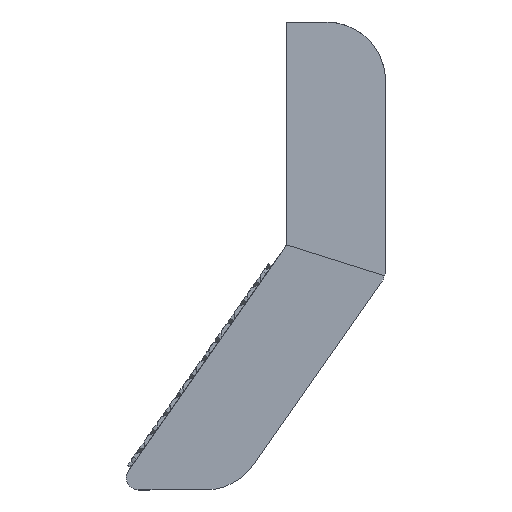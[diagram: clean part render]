
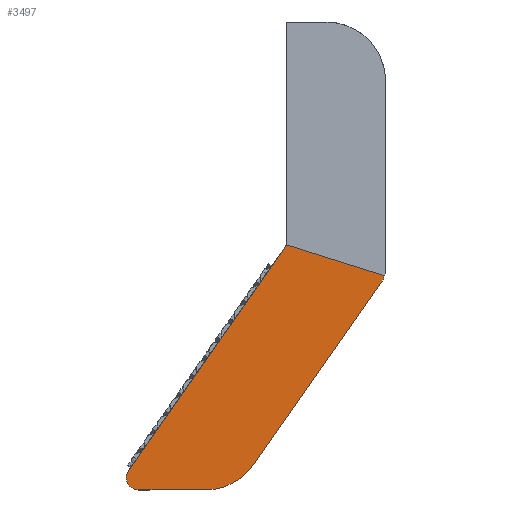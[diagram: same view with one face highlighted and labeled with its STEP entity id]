
A CAD part, left-side view. The second image highlights one B-rep face of the part: STEP entity #3497.
In plain terms, the highlighted planar face has unit normal (-0.999, -0.033, -0.023).
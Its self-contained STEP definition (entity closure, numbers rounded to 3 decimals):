
#36 = EDGE_CURVE ( 'NONE', #13042, #13123, #3158, .T. ) ;
#691 = CARTESIAN_POINT ( 'NONE',  ( -8.89, -15.225, -41.361 ) ) ;
#1274 = CARTESIAN_POINT ( 'NONE',  ( -9.399, 23.577, -74.676 ) ) ;
#1341 = DIRECTION ( 'NONE',  ( 0.033, -0.999, 0. ) ) ;
#1362 = CARTESIAN_POINT ( 'NONE',  ( -8.89, -15.225, -41.361 ) ) ;
#1385 = ORIENTED_EDGE ( 'NONE', *, *, #15113, .F. ) ;
#1728 = CARTESIAN_POINT ( 'NONE',  ( -9.525, 0.061, -35.626 ) ) ;
#1875 = ORIENTED_EDGE ( 'NONE', *, *, #10678, .F. ) ;
#1987 = LINE ( 'NONE', #13367, #2442 ) ;
#2082 = CARTESIAN_POINT ( 'NONE',  ( -9.399, 23.577, -74.676 ) ) ;
#2291 = VERTEX_POINT ( 'NONE', #15675 ) ;
#2442 = VECTOR ( 'NONE', #5008, 1000. ) ;
#2484 = EDGE_CURVE ( 'NONE', #17424, #4694, #1987, .T. ) ;
#2653 = CARTESIAN_POINT ( 'NONE',  ( -9.526, 0.037, -35.548 ) ) ;
#3158 =( BOUNDED_CURVE ( )  B_SPLINE_CURVE ( 3, ( #10948, #3732, #11009, #691 ),
 .UNSPECIFIED., .F., .F. ) 
 B_SPLINE_CURVE_WITH_KNOTS ( ( 4, 4 ),
 ( 5.978, 6.283 ),
 .UNSPECIFIED. ) 
 CURVE ( )  GEOMETRIC_REPRESENTATION_ITEM ( )  RATIONAL_B_SPLINE_CURVE ( ( 1., 0.992, 0.992, 1. ) ) 
 REPRESENTATION_ITEM ( '' )  );
#3220 = CARTESIAN_POINT ( 'NONE',  ( -9.399, 23.577, -74.676 ) ) ;
#3497 = ADVANCED_FACE ( 'NONE', ( #8715 ), #5661, .F. ) ;
#3581 = CARTESIAN_POINT ( 'NONE',  ( -9.46, 25.408, -74.676 ) ) ;
#3732 = CARTESIAN_POINT ( 'NONE',  ( -8.892, -15.554, -40.805 ) ) ;
#4188 = DIRECTION ( 'NONE',  ( 0.999, 0.033, 0.023 ) ) ;
#4454 = ORIENTED_EDGE ( 'NONE', *, *, #5288, .F. ) ;
#4624 =( BOUNDED_CURVE ( )  B_SPLINE_CURVE ( 3, ( #2082, #3581, #16139, #8078 ),
 .UNSPECIFIED., .F., .T. ) 
 B_SPLINE_CURVE_WITH_KNOTS ( ( 4, 4 ),
 ( 0.96, 3.142 ),
 .UNSPECIFIED. ) 
 CURVE ( )  GEOMETRIC_REPRESENTATION_ITEM ( )  RATIONAL_B_SPLINE_CURVE ( ( 1., 0.641, 0.641, 1. ) ) 
 REPRESENTATION_ITEM ( '' )  );
#4694 = VERTEX_POINT ( 'NONE', #5627 ) ;
#4769 = CARTESIAN_POINT ( 'NONE',  ( -9.525, 0.144, -35.765 ) ) ;
#5008 = DIRECTION ( 'NONE',  ( 0., 0.574, -0.819 ) ) ;
#5288 = EDGE_CURVE ( 'NONE', #9492, #13042, #16224, .T. ) ;
#5366 = CARTESIAN_POINT ( 'NONE',  ( -8.89, -15.225, -41.361 ) ) ;
#5627 = CARTESIAN_POINT ( 'NONE',  ( -9.525, 25.203, -71.553 ) ) ;
#5661 = PLANE ( 'NONE',  #12660 ) ;
#6237 = LINE ( 'NONE', #1274, #16676 ) ;
#6323 = CARTESIAN_POINT ( 'NONE',  ( -9.525, 0.144, -35.765 ) ) ;
#6362 = ORIENTED_EDGE ( 'NONE', *, *, #36, .F. ) ;
#6840 = CARTESIAN_POINT ( 'NONE',  ( -8.89, 5.259, -70.614 ) ) ;
#6990 = VECTOR ( 'NONE', #8749, 1000. ) ;
#6991 = EDGE_LOOP ( 'NONE', ( #4454, #12039, #12444, #1385, #9254, #1875, #13267, #6362 ) ) ;
#8078 = CARTESIAN_POINT ( 'NONE',  ( -9.525, 25.203, -71.553 ) ) ;
#8273 = CARTESIAN_POINT ( 'NONE',  ( -8.949, 9.89, -74.676 ) ) ;
#8715 = FACE_OUTER_BOUND ( 'NONE', #6991, .T. ) ;
#8749 = DIRECTION ( 'NONE',  ( 0., 0.574, -0.819 ) ) ;
#8948 = EDGE_CURVE ( 'NONE', #9492, #17424, #9407, .T. ) ;
#9254 = ORIENTED_EDGE ( 'NONE', *, *, #12468, .T. ) ;
#9407 =( BOUNDED_CURVE ( )  B_SPLINE_CURVE ( 3, ( #13176, #1728, #17095, #4769 ),
 .UNSPECIFIED., .F., .T. ) 
 B_SPLINE_CURVE_WITH_KNOTS ( ( 4, 4 ),
 ( 2.836, 3.142 ),
 .UNSPECIFIED. ) 
 CURVE ( )  GEOMETRIC_REPRESENTATION_ITEM ( )  RATIONAL_B_SPLINE_CURVE ( ( 1., 0.992, 0.992, 1. ) ) 
 REPRESENTATION_ITEM ( '' )  );
#9492 = VERTEX_POINT ( 'NONE', #15401 ) ;
#9546 = VECTOR ( 'NONE', #12680, 1000. ) ;
#10678 = EDGE_CURVE ( 'NONE', #2291, #13889, #14879, .T. ) ;
#10948 = CARTESIAN_POINT ( 'NONE',  ( -8.896, -15.652, -40.495 ) ) ;
#11009 = CARTESIAN_POINT ( 'NONE',  ( -8.89, -15.411, -41.096 ) ) ;
#11164 = LINE ( 'NONE', #1362, #6990 ) ;
#12039 = ORIENTED_EDGE ( 'NONE', *, *, #8948, .T. ) ;
#12444 = ORIENTED_EDGE ( 'NONE', *, *, #2484, .T. ) ;
#12468 = EDGE_CURVE ( 'NONE', #16759, #13889, #6237, .T. ) ;
#12660 = AXIS2_PLACEMENT_3D ( 'NONE', #16605, #4188, #14001 ) ;
#12680 = DIRECTION ( 'NONE',  ( 0.038, -0.953, -0.3 ) ) ;
#13042 = VERTEX_POINT ( 'NONE', #17567 ) ;
#13123 = VERTEX_POINT ( 'NONE', #5366 ) ;
#13176 = CARTESIAN_POINT ( 'NONE',  ( -9.526, 0.037, -35.548 ) ) ;
#13267 = ORIENTED_EDGE ( 'NONE', *, *, #14699, .F. ) ;
#13367 = CARTESIAN_POINT ( 'NONE',  ( -9.525, 0., -35.56 ) ) ;
#13655 = CARTESIAN_POINT ( 'NONE',  ( -8.89, 7.077, -73.212 ) ) ;
#13889 = VERTEX_POINT ( 'NONE', #17073 ) ;
#14001 = DIRECTION ( 'NONE',  ( -0.033, 0.999, 0. ) ) ;
#14699 = EDGE_CURVE ( 'NONE', #13123, #2291, #11164, .T. ) ;
#14879 =( BOUNDED_CURVE ( )  B_SPLINE_CURVE ( 3, ( #6840, #13655, #8273, #17651 ),
 .UNSPECIFIED., .F., .T. ) 
 B_SPLINE_CURVE_WITH_KNOTS ( ( 4, 4 ),
 ( 0., 0.96 ),
 .UNSPECIFIED. ) 
 CURVE ( )  GEOMETRIC_REPRESENTATION_ITEM ( )  RATIONAL_B_SPLINE_CURVE ( ( 1., 0.925, 0.925, 1. ) ) 
 REPRESENTATION_ITEM ( '' )  );
#15113 = EDGE_CURVE ( 'NONE', #16759, #4694, #4624, .T. ) ;
#15401 = CARTESIAN_POINT ( 'NONE',  ( -9.526, 0.037, -35.548 ) ) ;
#15675 = CARTESIAN_POINT ( 'NONE',  ( -8.89, 5.259, -70.614 ) ) ;
#16139 = CARTESIAN_POINT ( 'NONE',  ( -9.525, 26.253, -73.053 ) ) ;
#16224 = LINE ( 'NONE', #2653, #9546 ) ;
#16605 = CARTESIAN_POINT ( 'NONE',  ( -8.634, -22.173, -42.551 ) ) ;
#16676 = VECTOR ( 'NONE', #1341, 1000. ) ;
#16759 = VERTEX_POINT ( 'NONE', #3220 ) ;
#17073 = CARTESIAN_POINT ( 'NONE',  ( -9.053, 13.061, -74.676 ) ) ;
#17095 = CARTESIAN_POINT ( 'NONE',  ( -9.525, 0.097, -35.699 ) ) ;
#17424 = VERTEX_POINT ( 'NONE', #6323 ) ;
#17567 = CARTESIAN_POINT ( 'NONE',  ( -8.896, -15.652, -40.495 ) ) ;
#17651 = CARTESIAN_POINT ( 'NONE',  ( -9.053, 13.061, -74.676 ) ) ;
